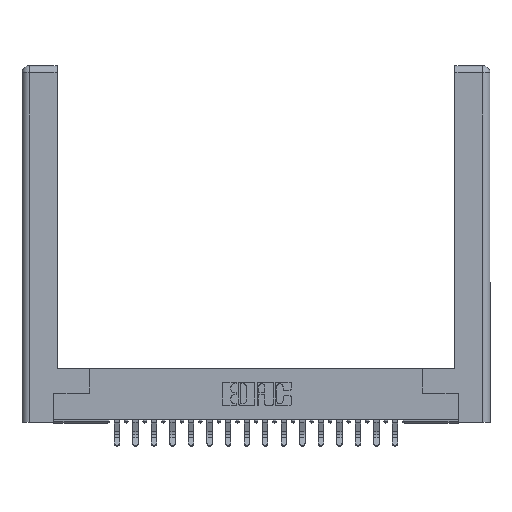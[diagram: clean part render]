
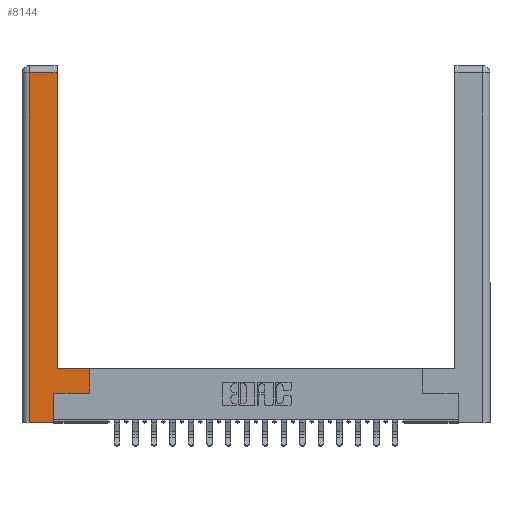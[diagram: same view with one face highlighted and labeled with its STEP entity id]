
A CAD part, top view. The second image highlights one B-rep face of the part: STEP entity #8144.
In plain terms, the highlighted planar face has unit normal (0, 0, 1).
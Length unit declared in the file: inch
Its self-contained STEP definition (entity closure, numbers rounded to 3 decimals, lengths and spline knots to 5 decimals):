
#340 = VECTOR ( 'NONE', #3053, 39.37008 ) ;
#477 = DIRECTION ( 'NONE',  ( 0., 1., 0. ) ) ;
#480 = ORIENTED_EDGE ( 'NONE', *, *, #3120, .T. ) ;
#849 = ORIENTED_EDGE ( 'NONE', *, *, #2456, .T. ) ;
#929 = CARTESIAN_POINT ( 'NONE',  ( 0.0615, 2.94, 0. ) ) ;
#1295 = ORIENTED_EDGE ( 'NONE', *, *, #19247, .T. ) ;
#2059 = PLANE ( 'NONE',  #13410 ) ;
#2285 = EDGE_LOOP ( 'NONE', ( #480, #4034, #9142, #849, #11929, #1295, #15411, #11534 ) ) ;
#2430 = VERTEX_POINT ( 'NONE', #8374 ) ;
#2456 = EDGE_CURVE ( 'NONE', #23093, #22455, #8853, .T. ) ;
#2474 = CARTESIAN_POINT ( 'NONE',  ( 0.265, 0., 0. ) ) ;
#2509 = VERTEX_POINT ( 'NONE', #3860 ) ;
#2783 = EDGE_CURVE ( 'NONE', #2509, #23093, #10776, .T. ) ;
#3053 = DIRECTION ( 'NONE',  ( -1., 0., 0. ) ) ;
#3120 = EDGE_CURVE ( 'NONE', #14186, #2430, #9110, .T. ) ;
#3529 = LINE ( 'NONE', #5667, #22693 ) ;
#3690 = EDGE_CURVE ( 'NONE', #22455, #12067, #15510, .T. ) ;
#3860 = CARTESIAN_POINT ( 'NONE',  ( 0.0615, 2.94, 0. ) ) ;
#4034 = ORIENTED_EDGE ( 'NONE', *, *, #11975, .T. ) ;
#4192 = CARTESIAN_POINT ( 'NONE',  ( 0.0615, 0., 0. ) ) ;
#5587 = DIRECTION ( 'NONE',  ( -1., 0., 0. ) ) ;
#5667 = CARTESIAN_POINT ( 'NONE',  ( 0.565, 0.245, 0. ) ) ;
#5736 = DIRECTION ( 'NONE',  ( 0., 0., -1. ) ) ;
#6274 = EDGE_CURVE ( 'NONE', #17046, #14186, #10023, .T. ) ;
#6898 = CARTESIAN_POINT ( 'NONE',  ( 0.265, 0.245, 0. ) ) ;
#7703 = VECTOR ( 'NONE', #20440, 39.37008 ) ;
#7921 = VECTOR ( 'NONE', #18811, 39.37008 ) ;
#7966 = CARTESIAN_POINT ( 'NONE',  ( 0.295, 0.45, 0. ) ) ;
#8144 = ADVANCED_FACE ( 'NONE', ( #10603 ), #2059, .F. ) ;
#8374 = CARTESIAN_POINT ( 'NONE',  ( 0.295, 2.94, 0. ) ) ;
#8626 = CARTESIAN_POINT ( 'NONE',  ( 0.565, 0.45, 0. ) ) ;
#8853 = LINE ( 'NONE', #20640, #17542 ) ;
#9110 = LINE ( 'NONE', #11171, #16414 ) ;
#9142 = ORIENTED_EDGE ( 'NONE', *, *, #2783, .T. ) ;
#9754 = CARTESIAN_POINT ( 'NONE',  ( 0.265, 0.245, 0. ) ) ;
#10023 = LINE ( 'NONE', #19151, #20794 ) ;
#10095 = DIRECTION ( 'NONE',  ( 1., 0., 0. ) ) ;
#10603 = FACE_OUTER_BOUND ( 'NONE', #2285, .T. ) ;
#10776 = LINE ( 'NONE', #20369, #7703 ) ;
#11171 = CARTESIAN_POINT ( 'NONE',  ( 0.295, 3., 0. ) ) ;
#11275 = LINE ( 'NONE', #12565, #15185 ) ;
#11534 = ORIENTED_EDGE ( 'NONE', *, *, #6274, .T. ) ;
#11929 = ORIENTED_EDGE ( 'NONE', *, *, #3690, .T. ) ;
#11975 = EDGE_CURVE ( 'NONE', #2430, #2509, #13263, .T. ) ;
#12067 = VERTEX_POINT ( 'NONE', #6898 ) ;
#12565 = CARTESIAN_POINT ( 'NONE',  ( 0.565, 0.45, 0. ) ) ;
#13263 = LINE ( 'NONE', #929, #340 ) ;
#13410 = AXIS2_PLACEMENT_3D ( 'NONE', #14651, #5736, #5587 ) ;
#14186 = VERTEX_POINT ( 'NONE', #7966 ) ;
#14651 = CARTESIAN_POINT ( 'NONE',  ( 0., 0., 0. ) ) ;
#15185 = VECTOR ( 'NONE', #21684, 39.37008 ) ;
#15411 = ORIENTED_EDGE ( 'NONE', *, *, #16156, .T. ) ;
#15510 = LINE ( 'NONE', #9754, #7921 ) ;
#15520 = CARTESIAN_POINT ( 'NONE',  ( 0.565, 0.245, 0. ) ) ;
#15864 = VERTEX_POINT ( 'NONE', #15520 ) ;
#16156 = EDGE_CURVE ( 'NONE', #15864, #17046, #11275, .T. ) ;
#16414 = VECTOR ( 'NONE', #477, 39.37008 ) ;
#17046 = VERTEX_POINT ( 'NONE', #8626 ) ;
#17542 = VECTOR ( 'NONE', #10095, 39.37008 ) ;
#18811 = DIRECTION ( 'NONE',  ( 0., 1., 0. ) ) ;
#19151 = CARTESIAN_POINT ( 'NONE',  ( 0.295, 0.45, 0. ) ) ;
#19247 = EDGE_CURVE ( 'NONE', #12067, #15864, #3529, .T. ) ;
#20012 = DIRECTION ( 'NONE',  ( 1., 0., 0. ) ) ;
#20369 = CARTESIAN_POINT ( 'NONE',  ( 0.0615, 0., 0. ) ) ;
#20440 = DIRECTION ( 'NONE',  ( 0., -1., 0. ) ) ;
#20640 = CARTESIAN_POINT ( 'NONE',  ( 0.265, 0., 0. ) ) ;
#20794 = VECTOR ( 'NONE', #22684, 39.37008 ) ;
#21684 = DIRECTION ( 'NONE',  ( 0., 1., 0. ) ) ;
#22455 = VERTEX_POINT ( 'NONE', #2474 ) ;
#22684 = DIRECTION ( 'NONE',  ( -1., 0., 0. ) ) ;
#22693 = VECTOR ( 'NONE', #20012, 39.37008 ) ;
#23093 = VERTEX_POINT ( 'NONE', #4192 ) ;
